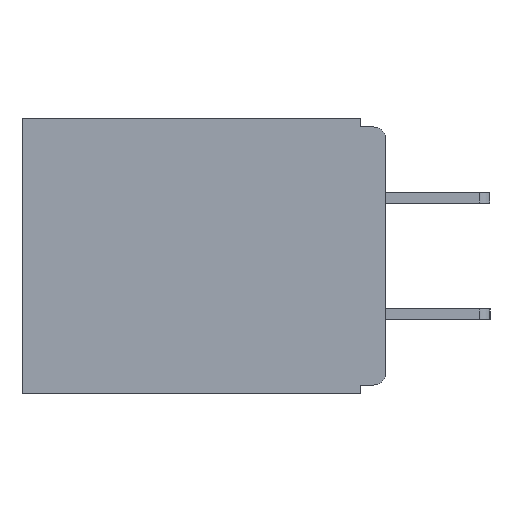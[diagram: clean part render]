
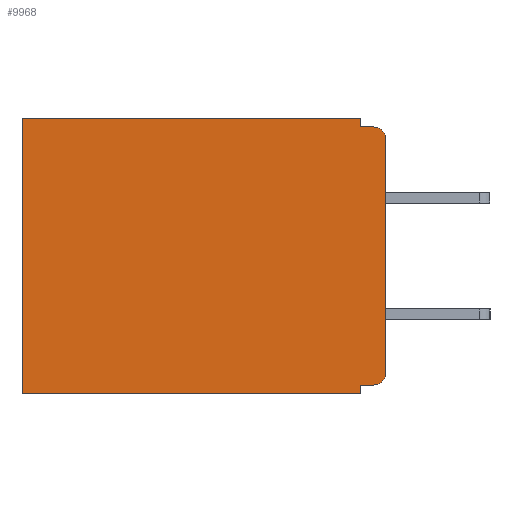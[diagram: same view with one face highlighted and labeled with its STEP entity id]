
A CAD part, left-side view. The second image highlights one B-rep face of the part: STEP entity #9968.
In plain terms, the highlighted planar face has unit normal (-1, 0, 0).
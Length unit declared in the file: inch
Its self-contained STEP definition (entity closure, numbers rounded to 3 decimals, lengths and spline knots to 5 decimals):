
#44 = ORIENTED_EDGE ( 'NONE', *, *, #11914, .T. ) ;
#261 = DIRECTION ( 'NONE',  ( 0., 0., -1. ) ) ;
#523 = ORIENTED_EDGE ( 'NONE', *, *, #10686, .T. ) ;
#537 = CARTESIAN_POINT ( 'NONE',  ( 0.3, 0.031, -0.33 ) ) ;
#665 = EDGE_CURVE ( 'NONE', #10745, #7772, #19117, .T. ) ;
#786 = PLANE ( 'NONE',  #1874 ) ;
#1096 = CARTESIAN_POINT ( 'NONE',  ( 0.3, 0.015, -0.025 ) ) ;
#1157 = DIRECTION ( 'NONE',  ( 0., 0., -1. ) ) ;
#1161 = VERTEX_POINT ( 'NONE', #5222 ) ;
#1276 = ORIENTED_EDGE ( 'NONE', *, *, #665, .T. ) ;
#1425 = CARTESIAN_POINT ( 'NONE',  ( 0.3, 0.031, 0. ) ) ;
#1874 = AXIS2_PLACEMENT_3D ( 'NONE', #14234, #11324, #2355 ) ;
#1982 = EDGE_CURVE ( 'NONE', #1161, #14170, #19066, .T. ) ;
#2225 = VECTOR ( 'NONE', #1157, 39.37008 ) ;
#2268 = VERTEX_POINT ( 'NONE', #17238 ) ;
#2355 = DIRECTION ( 'NONE',  ( 0., 0., -1. ) ) ;
#2646 = DIRECTION ( 'NONE',  ( 0., 0., -1. ) ) ;
#2686 = LINE ( 'NONE', #4257, #2225 ) ;
#2890 = AXIS2_PLACEMENT_3D ( 'NONE', #15847, #6986, #17329 ) ;
#2900 = VECTOR ( 'NONE', #15276, 39.37008 ) ;
#3408 = CIRCLE ( 'NONE', #2890, 0.015 ) ;
#3671 = CARTESIAN_POINT ( 'NONE',  ( 0.3, 0.031, -0.32 ) ) ;
#3733 = VERTEX_POINT ( 'NONE', #18547 ) ;
#4257 = CARTESIAN_POINT ( 'NONE',  ( 0.3, 0., -0.33 ) ) ;
#4517 = LINE ( 'NONE', #17397, #8051 ) ;
#4819 = DIRECTION ( 'NONE',  ( 0., 1., 0. ) ) ;
#5222 = CARTESIAN_POINT ( 'NONE',  ( 0.3, 0.015, -0.32 ) ) ;
#5645 = LINE ( 'NONE', #7889, #9167 ) ;
#6070 = ORIENTED_EDGE ( 'NONE', *, *, #6725, .F. ) ;
#6725 = EDGE_CURVE ( 'NONE', #2268, #7772, #11715, .T. ) ;
#6986 = DIRECTION ( 'NONE',  ( -1., 0., 0. ) ) ;
#7063 = DIRECTION ( 'NONE',  ( 0., 1., 0. ) ) ;
#7512 = EDGE_CURVE ( 'NONE', #7532, #3733, #13531, .T. ) ;
#7532 = VERTEX_POINT ( 'NONE', #12881 ) ;
#7692 = EDGE_LOOP ( 'NONE', ( #17514, #523, #15909, #8589, #44, #1276, #6070, #15552, #14176, #17826 ) ) ;
#7772 = VERTEX_POINT ( 'NONE', #18785 ) ;
#7802 = VECTOR ( 'NONE', #9966, 39.37008 ) ;
#7889 = CARTESIAN_POINT ( 'NONE',  ( 0.3, 0.031, 0. ) ) ;
#8051 = VECTOR ( 'NONE', #7063, 39.37008 ) ;
#8338 = VERTEX_POINT ( 'NONE', #1425 ) ;
#8589 = ORIENTED_EDGE ( 'NONE', *, *, #17582, .F. ) ;
#9167 = VECTOR ( 'NONE', #261, 39.37008 ) ;
#9738 = CIRCLE ( 'NONE', #11184, 0.015 ) ;
#9966 = DIRECTION ( 'NONE',  ( 0., 1., 0. ) ) ;
#9968 = ADVANCED_FACE ( 'NONE', ( #19138 ), #786, .F. ) ;
#9992 = EDGE_CURVE ( 'NONE', #1161, #12494, #3408, .T. ) ;
#10537 = CARTESIAN_POINT ( 'NONE',  ( 0.3, 0., -0.33 ) ) ;
#10686 = EDGE_CURVE ( 'NONE', #11204, #3733, #9738, .T. ) ;
#10745 = VERTEX_POINT ( 'NONE', #11686 ) ;
#11184 = AXIS2_PLACEMENT_3D ( 'NONE', #1096, #11625, #2646 ) ;
#11204 = VERTEX_POINT ( 'NONE', #15738 ) ;
#11324 = DIRECTION ( 'NONE',  ( 1., 0., 0. ) ) ;
#11471 = LINE ( 'NONE', #537, #14948 ) ;
#11625 = DIRECTION ( 'NONE',  ( -1., 0., 0. ) ) ;
#11686 = CARTESIAN_POINT ( 'NONE',  ( 0.3, 0.437, 0. ) ) ;
#11715 = LINE ( 'NONE', #10537, #7802 ) ;
#11914 = EDGE_CURVE ( 'NONE', #8338, #10745, #4517, .T. ) ;
#12494 = VERTEX_POINT ( 'NONE', #18931 ) ;
#12606 = DIRECTION ( 'NONE',  ( 0., 0., -1. ) ) ;
#12881 = CARTESIAN_POINT ( 'NONE',  ( 0.3, 0.031, -0.01 ) ) ;
#13504 = EDGE_CURVE ( 'NONE', #14170, #2268, #11471, .T. ) ;
#13531 = LINE ( 'NONE', #14714, #17016 ) ;
#14121 = CARTESIAN_POINT ( 'NONE',  ( 0.3, 0.437, -0.33 ) ) ;
#14170 = VERTEX_POINT ( 'NONE', #3671 ) ;
#14176 = ORIENTED_EDGE ( 'NONE', *, *, #1982, .F. ) ;
#14234 = CARTESIAN_POINT ( 'NONE',  ( 0.3, 0., -0.33 ) ) ;
#14267 = DIRECTION ( 'NONE',  ( 0., -1., 0. ) ) ;
#14714 = CARTESIAN_POINT ( 'NONE',  ( 0.3, 0., -0.01 ) ) ;
#14948 = VECTOR ( 'NONE', #12606, 39.37008 ) ;
#15222 = VECTOR ( 'NONE', #4819, 39.37008 ) ;
#15276 = DIRECTION ( 'NONE',  ( 0., 0., -1. ) ) ;
#15552 = ORIENTED_EDGE ( 'NONE', *, *, #13504, .F. ) ;
#15738 = CARTESIAN_POINT ( 'NONE',  ( 0.3, 0., -0.025 ) ) ;
#15847 = CARTESIAN_POINT ( 'NONE',  ( 0.3, 0.015, -0.305 ) ) ;
#15909 = ORIENTED_EDGE ( 'NONE', *, *, #7512, .F. ) ;
#17016 = VECTOR ( 'NONE', #14267, 39.37008 ) ;
#17238 = CARTESIAN_POINT ( 'NONE',  ( 0.3, 0.031, -0.33 ) ) ;
#17262 = CARTESIAN_POINT ( 'NONE',  ( 0.3, 0., -0.32 ) ) ;
#17329 = DIRECTION ( 'NONE',  ( 0., 0., -1. ) ) ;
#17397 = CARTESIAN_POINT ( 'NONE',  ( 0.3, 0., 0. ) ) ;
#17514 = ORIENTED_EDGE ( 'NONE', *, *, #19193, .F. ) ;
#17582 = EDGE_CURVE ( 'NONE', #8338, #7532, #5645, .T. ) ;
#17826 = ORIENTED_EDGE ( 'NONE', *, *, #9992, .T. ) ;
#18547 = CARTESIAN_POINT ( 'NONE',  ( 0.3, 0.015, -0.01 ) ) ;
#18785 = CARTESIAN_POINT ( 'NONE',  ( 0.3, 0.437, -0.33 ) ) ;
#18931 = CARTESIAN_POINT ( 'NONE',  ( 0.3, 0., -0.305 ) ) ;
#19066 = LINE ( 'NONE', #17262, #15222 ) ;
#19117 = LINE ( 'NONE', #14121, #2900 ) ;
#19138 = FACE_OUTER_BOUND ( 'NONE', #7692, .T. ) ;
#19193 = EDGE_CURVE ( 'NONE', #11204, #12494, #2686, .T. ) ;
